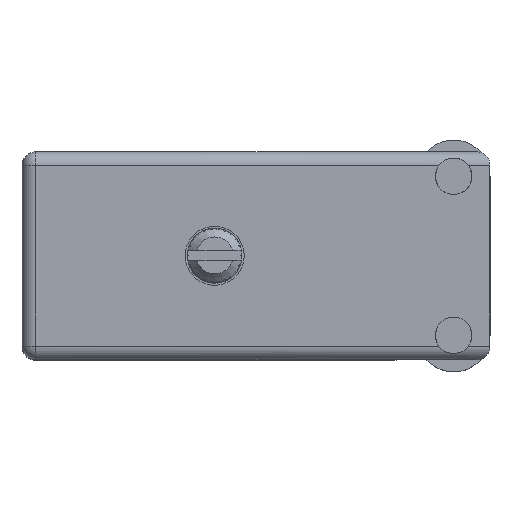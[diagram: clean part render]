
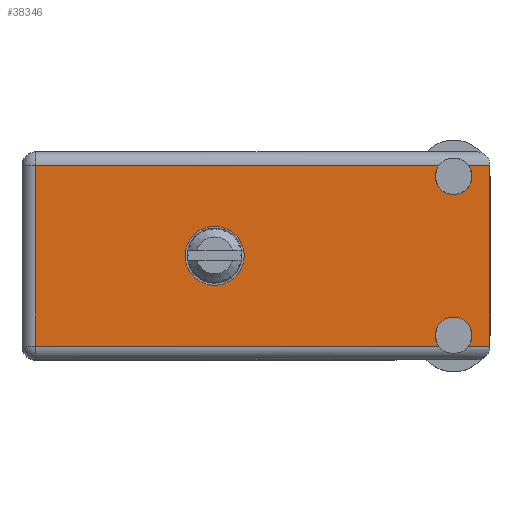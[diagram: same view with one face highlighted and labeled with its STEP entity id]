
A CAD part, top view. The second image highlights one B-rep face of the part: STEP entity #38346.
In plain terms, the highlighted face is planar.
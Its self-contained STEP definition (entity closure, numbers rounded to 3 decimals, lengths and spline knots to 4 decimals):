
#178 = ORIENTED_EDGE ( 'NONE', *, *, #49724, .T. ) ;
#2143 = EDGE_CURVE ( 'NONE', #33673, #108215, #30285, .T. ) ;
#3432 = CARTESIAN_POINT ( 'NONE',  ( 0.047, 0.906, -0.047 ) ) ;
#3690 = EDGE_CURVE ( 'NONE', #121549, #185090, #123717, .T. ) ;
#6121 = DIRECTION ( 'NONE',  ( 0., 0., 1. ) ) ;
#6758 = VERTEX_POINT ( 'NONE', #145573 ) ;
#10384 = EDGE_CURVE ( 'NONE', #78939, #28239, #112310, .T. ) ;
#10671 = CARTESIAN_POINT ( 'NONE',  ( 1.609, 0.906, -0.668 ) ) ;
#18233 = EDGE_CURVE ( 'NONE', #108215, #157868, #70648, .T. ) ;
#18876 = DIRECTION ( 'NONE',  ( 0., 1., 0. ) ) ;
#20509 = DIRECTION ( 'NONE',  ( 0., 0., 1. ) ) ;
#24052 = EDGE_LOOP ( 'NONE', ( #151623, #108922, #33440, #178, #63755, #88778, #48545, #27855, #44073, #118383 ) ) ;
#25170 = ORIENTED_EDGE ( 'NONE', *, *, #162907, .F. ) ;
#27855 = ORIENTED_EDGE ( 'NONE', *, *, #181456, .F. ) ;
#28239 = VERTEX_POINT ( 'NONE', #45704 ) ;
#30104 = VECTOR ( 'NONE', #63258, 39.3701 ) ;
#30285 = LINE ( 'NONE', #111301, #80556 ) ;
#31613 = CARTESIAN_POINT ( 'NONE',  ( 1.609, 0.906, -0.047 ) ) ;
#33341 = ORIENTED_EDGE ( 'NONE', *, *, #91784, .F. ) ;
#33440 = ORIENTED_EDGE ( 'NONE', *, *, #10384, .F. ) ;
#33673 = VERTEX_POINT ( 'NONE', #197022 ) ;
#34098 = DIRECTION ( 'NONE',  ( 0., 0., 1. ) ) ;
#36310 = DIRECTION ( 'NONE',  ( 0., 1., 0. ) ) ;
#38346 = ADVANCED_FACE ( 'NONE', ( #115967, #50762 ), #191414, .T. ) ;
#43855 = CARTESIAN_POINT ( 'NONE',  ( 1.484, 0.906, -0.631 ) ) ;
#44073 = ORIENTED_EDGE ( 'NONE', *, *, #117015, .T. ) ;
#44120 = DIRECTION ( 'NONE',  ( 1., 0., 0. ) ) ;
#45704 = CARTESIAN_POINT ( 'NONE',  ( 1.484, 0.906, -0.1465 ) ) ;
#46918 = DIRECTION ( 'NONE',  ( 0., 1., 0. ) ) ;
#48545 = ORIENTED_EDGE ( 'NONE', *, *, #97609, .F. ) ;
#49137 = CARTESIAN_POINT ( 'NONE',  ( 1.609, 0.906, 0. ) ) ;
#49724 = EDGE_CURVE ( 'NONE', #78939, #185090, #113075, .T. ) ;
#49804 = DIRECTION ( 'NONE',  ( -1., 0., 0. ) ) ;
#50762 = FACE_OUTER_BOUND ( 'NONE', #24052, .T. ) ;
#52011 = CARTESIAN_POINT ( 'NONE',  ( 1.4336, 0.906, -0.047 ) ) ;
#56231 = VECTOR ( 'NONE', #49804, 39.3701 ) ;
#56664 = VECTOR ( 'NONE', #159795, 39.3701 ) ;
#58010 = DIRECTION ( 'NONE',  ( 0., 1., 0. ) ) ;
#58709 = LINE ( 'NONE', #141833, #56231 ) ;
#63258 = DIRECTION ( 'NONE',  ( 0., 0., 1. ) ) ;
#63755 = ORIENTED_EDGE ( 'NONE', *, *, #3690, .F. ) ;
#64559 = CARTESIAN_POINT ( 'NONE',  ( 1.484, 0.906, -0.084 ) ) ;
#66839 = CIRCLE ( 'NONE', #180058, 0.0625 ) ;
#70116 = VERTEX_POINT ( 'NONE', #162649 ) ;
#70648 = LINE ( 'NONE', #31613, #168957 ) ;
#71113 = LINE ( 'NONE', #97396, #56664 ) ;
#73169 = CIRCLE ( 'NONE', #185302, 0.0625 ) ;
#75970 = CARTESIAN_POINT ( 'NONE',  ( 1.609, 0.906, -0.047 ) ) ;
#76721 = AXIS2_PLACEMENT_3D ( 'NONE', #160094, #112461, #20509 ) ;
#78939 = VERTEX_POINT ( 'NONE', #129799 ) ;
#80556 = VECTOR ( 'NONE', #34098, 39.3701 ) ;
#82786 = DIRECTION ( 'NONE',  ( 0., 1., 0. ) ) ;
#86998 = DIRECTION ( 'NONE',  ( 0., 1., 0. ) ) ;
#87107 = AXIS2_PLACEMENT_3D ( 'NONE', #64559, #18876, #140454 ) ;
#88044 = CARTESIAN_POINT ( 'NONE',  ( 1.5344, 0.906, -0.668 ) ) ;
#88778 = ORIENTED_EDGE ( 'NONE', *, *, #186957, .T. ) ;
#89490 = CIRCLE ( 'NONE', #76721, 0.1015 ) ;
#91784 = EDGE_CURVE ( 'NONE', #6758, #93583, #89490, .T. ) ;
#93583 = VERTEX_POINT ( 'NONE', #170824 ) ;
#97396 = CARTESIAN_POINT ( 'NONE',  ( 0., 0.906, -0.668 ) ) ;
#97609 = EDGE_CURVE ( 'NONE', #169122, #174336, #139074, .T. ) ;
#108215 = VERTEX_POINT ( 'NONE', #3432 ) ;
#108922 = ORIENTED_EDGE ( 'NONE', *, *, #138098, .F. ) ;
#111301 = CARTESIAN_POINT ( 'NONE',  ( 0.047, 0.906, -0.715 ) ) ;
#112310 = CIRCLE ( 'NONE', #87107, 0.0625 ) ;
#112461 = DIRECTION ( 'NONE',  ( 0., 1., 0. ) ) ;
#113075 = LINE ( 'NONE', #130827, #153890 ) ;
#115967 = FACE_BOUND ( 'NONE', #143219, .T. ) ;
#117015 = EDGE_CURVE ( 'NONE', #70116, #33673, #71113, .T. ) ;
#118383 = ORIENTED_EDGE ( 'NONE', *, *, #2143, .T. ) ;
#119041 = DIRECTION ( 'NONE',  ( 0., 0., 1. ) ) ;
#121549 = VERTEX_POINT ( 'NONE', #10671 ) ;
#123717 = LINE ( 'NONE', #49137, #30104 ) ;
#124114 = CARTESIAN_POINT ( 'NONE',  ( 1.484, 0.906, -0.084 ) ) ;
#129068 = AXIS2_PLACEMENT_3D ( 'NONE', #173863, #36310, #6121 ) ;
#129799 = CARTESIAN_POINT ( 'NONE',  ( 1.5344, 0.906, -0.047 ) ) ;
#130424 = CARTESIAN_POINT ( 'NONE',  ( 0., 0.906, -0.715 ) ) ;
#130827 = CARTESIAN_POINT ( 'NONE',  ( 1.609, 0.906, -0.047 ) ) ;
#131937 = CIRCLE ( 'NONE', #135792, 0.1015 ) ;
#135792 = AXIS2_PLACEMENT_3D ( 'NONE', #178911, #86998, #194304 ) ;
#138098 = EDGE_CURVE ( 'NONE', #28239, #157868, #73169, .T. ) ;
#139074 = CIRCLE ( 'NONE', #129068, 0.0625 ) ;
#140454 = DIRECTION ( 'NONE',  ( 0., 0., 1. ) ) ;
#141833 = CARTESIAN_POINT ( 'NONE',  ( 0., 0.906, -0.668 ) ) ;
#143219 = EDGE_LOOP ( 'NONE', ( #25170, #33341 ) ) ;
#145573 = CARTESIAN_POINT ( 'NONE',  ( 0.6625, 0.906, -0.459 ) ) ;
#151623 = ORIENTED_EDGE ( 'NONE', *, *, #18233, .T. ) ;
#153611 = DIRECTION ( 'NONE',  ( 0., 0., 1. ) ) ;
#153890 = VECTOR ( 'NONE', #44120, 39.3701 ) ;
#157868 = VERTEX_POINT ( 'NONE', #52011 ) ;
#159795 = DIRECTION ( 'NONE',  ( -1., 0., 0. ) ) ;
#160094 = CARTESIAN_POINT ( 'NONE',  ( 0.6625, 0.906, -0.3575 ) ) ;
#162649 = CARTESIAN_POINT ( 'NONE',  ( 1.4336, 0.906, -0.668 ) ) ;
#162907 = EDGE_CURVE ( 'NONE', #93583, #6758, #131937, .T. ) ;
#168957 = VECTOR ( 'NONE', #169858, 39.3701 ) ;
#169122 = VERTEX_POINT ( 'NONE', #192001 ) ;
#169858 = DIRECTION ( 'NONE',  ( 1., 0., 0. ) ) ;
#170824 = CARTESIAN_POINT ( 'NONE',  ( 0.6625, 0.906, -0.256 ) ) ;
#173863 = CARTESIAN_POINT ( 'NONE',  ( 1.484, 0.906, -0.631 ) ) ;
#173993 = DIRECTION ( 'NONE',  ( 0., 0., 1. ) ) ;
#174336 = VERTEX_POINT ( 'NONE', #88044 ) ;
#178911 = CARTESIAN_POINT ( 'NONE',  ( 0.6625, 0.906, -0.3575 ) ) ;
#180058 = AXIS2_PLACEMENT_3D ( 'NONE', #43855, #58010, #119041 ) ;
#181456 = EDGE_CURVE ( 'NONE', #70116, #169122, #66839, .T. ) ;
#185090 = VERTEX_POINT ( 'NONE', #75970 ) ;
#185302 = AXIS2_PLACEMENT_3D ( 'NONE', #124114, #46918, #153611 ) ;
#186957 = EDGE_CURVE ( 'NONE', #121549, #174336, #58709, .T. ) ;
#188902 = AXIS2_PLACEMENT_3D ( 'NONE', #130424, #82786, #173993 ) ;
#191414 = PLANE ( 'NONE',  #188902 ) ;
#192001 = CARTESIAN_POINT ( 'NONE',  ( 1.484, 0.906, -0.5685 ) ) ;
#194304 = DIRECTION ( 'NONE',  ( 0., 0., 1. ) ) ;
#197022 = CARTESIAN_POINT ( 'NONE',  ( 0.047, 0.906, -0.668 ) ) ;
